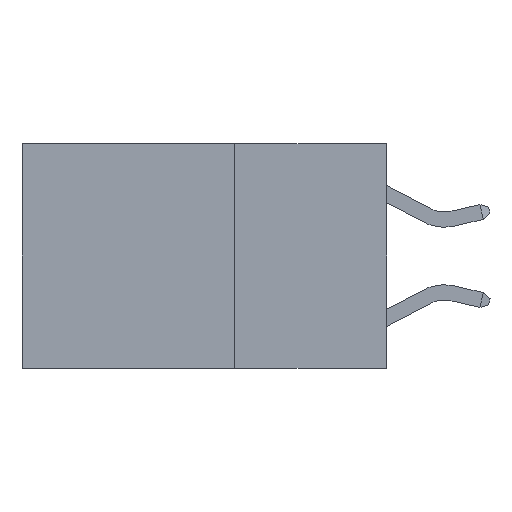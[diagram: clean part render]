
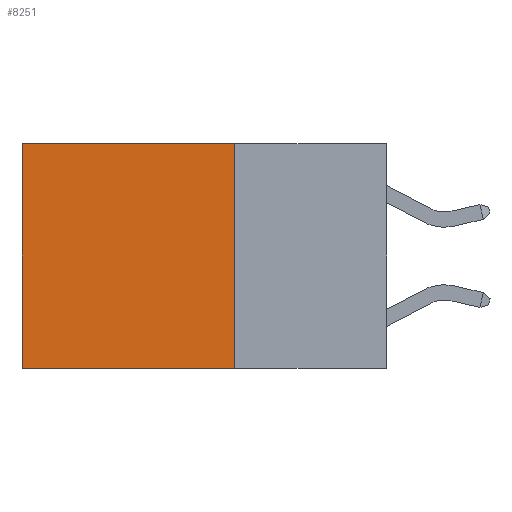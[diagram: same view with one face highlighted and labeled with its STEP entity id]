
A CAD part, left-side view. The second image highlights one B-rep face of the part: STEP entity #8251.
In plain terms, the highlighted planar face has unit normal (-1, 0, 0).
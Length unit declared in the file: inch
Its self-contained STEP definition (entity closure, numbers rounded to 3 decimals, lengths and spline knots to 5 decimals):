
#33 = VERTEX_POINT ( 'NONE', #9156 ) ;
#71 = PLANE ( 'NONE',  #6534 ) ;
#130 = CARTESIAN_POINT ( 'NONE',  ( 0.2625, 0.25, 0. ) ) ;
#200 = LINE ( 'NONE', #9756, #9747 ) ;
#265 = VECTOR ( 'NONE', #3887, 39.37008 ) ;
#308 = VERTEX_POINT ( 'NONE', #8610 ) ;
#318 = VERTEX_POINT ( 'NONE', #9546 ) ;
#1021 = CARTESIAN_POINT ( 'NONE',  ( 0.2625, 0.25, 0. ) ) ;
#1590 = DIRECTION ( 'NONE',  ( 0., 0., -1. ) ) ;
#1696 = ORIENTED_EDGE ( 'NONE', *, *, #11021, .T. ) ;
#1964 = DIRECTION ( 'NONE',  ( 1., 0., 0. ) ) ;
#2746 = LINE ( 'NONE', #7554, #265 ) ;
#2879 = VECTOR ( 'NONE', #1590, 39.37008 ) ;
#2899 = CARTESIAN_POINT ( 'NONE',  ( 0.2625, 0.25, 0. ) ) ;
#3861 = ORIENTED_EDGE ( 'NONE', *, *, #6993, .F. ) ;
#3887 = DIRECTION ( 'NONE',  ( 0., 0., -1. ) ) ;
#4229 = DIRECTION ( 'NONE',  ( 0., 1., 0. ) ) ;
#4322 = VECTOR ( 'NONE', #5662, 39.37008 ) ;
#5662 = DIRECTION ( 'NONE',  ( 0., 1., 0. ) ) ;
#6534 = AXIS2_PLACEMENT_3D ( 'NONE', #1021, #1964, #8385 ) ;
#6792 = LINE ( 'NONE', #2899, #4322 ) ;
#6993 = EDGE_CURVE ( 'NONE', #308, #33, #200, .T. ) ;
#7123 = CARTESIAN_POINT ( 'NONE',  ( 0.2625, 0.25, 0. ) ) ;
#7183 = EDGE_LOOP ( 'NONE', ( #8455, #3861, #8754, #1696 ) ) ;
#7554 = CARTESIAN_POINT ( 'NONE',  ( 0.2625, 0.6, 0. ) ) ;
#8109 = FACE_OUTER_BOUND ( 'NONE', #7183, .T. ) ;
#8251 = ADVANCED_FACE ( 'NONE', ( #8109 ), #71, .F. ) ;
#8385 = DIRECTION ( 'NONE',  ( 0., 0., -1. ) ) ;
#8455 = ORIENTED_EDGE ( 'NONE', *, *, #10231, .T. ) ;
#8610 = CARTESIAN_POINT ( 'NONE',  ( 0.2625, 0.25, -0.37 ) ) ;
#8754 = ORIENTED_EDGE ( 'NONE', *, *, #10443, .F. ) ;
#9156 = CARTESIAN_POINT ( 'NONE',  ( 0.2625, 0.6, -0.37 ) ) ;
#9546 = CARTESIAN_POINT ( 'NONE',  ( 0.2625, 0.6, 0. ) ) ;
#9747 = VECTOR ( 'NONE', #4229, 39.37008 ) ;
#9756 = CARTESIAN_POINT ( 'NONE',  ( 0.2625, 0.25, -0.37 ) ) ;
#10231 = EDGE_CURVE ( 'NONE', #318, #33, #2746, .T. ) ;
#10235 = LINE ( 'NONE', #7123, #2879 ) ;
#10443 = EDGE_CURVE ( 'NONE', #11027, #308, #10235, .T. ) ;
#11021 = EDGE_CURVE ( 'NONE', #11027, #318, #6792, .T. ) ;
#11027 = VERTEX_POINT ( 'NONE', #130 ) ;
